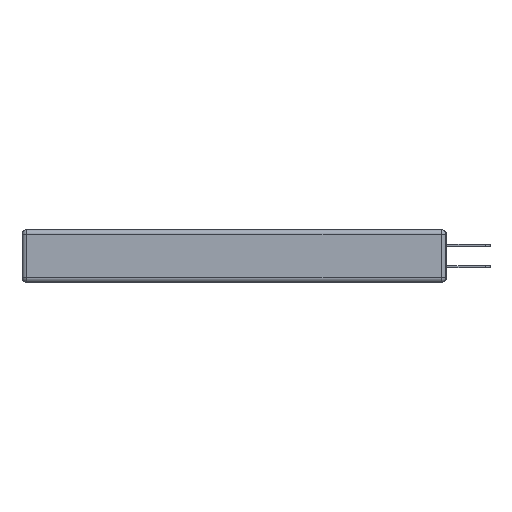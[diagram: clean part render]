
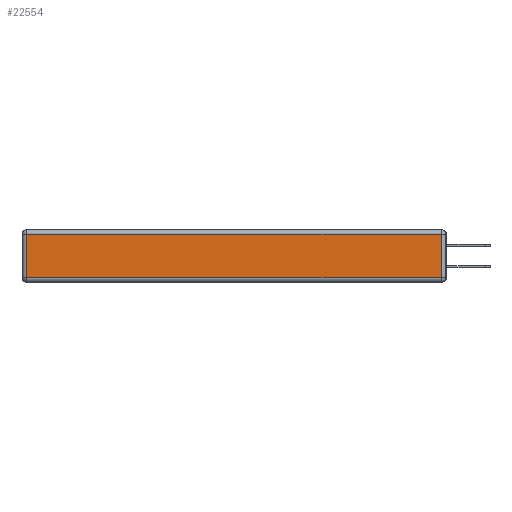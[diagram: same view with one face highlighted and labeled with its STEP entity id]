
A CAD part, left-side view. The second image highlights one B-rep face of the part: STEP entity #22554.
In plain terms, the highlighted planar face has unit normal (-1, 0, 0).
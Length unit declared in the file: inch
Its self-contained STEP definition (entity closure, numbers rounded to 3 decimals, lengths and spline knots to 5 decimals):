
#758 = DIRECTION ( 'NONE',  ( 0., -1., 0. ) ) ;
#1294 = CARTESIAN_POINT ( 'NONE',  ( 0., 2.72, -0.343 ) ) ;
#2915 = VERTEX_POINT ( 'NONE', #11813 ) ;
#3330 = CARTESIAN_POINT ( 'NONE',  ( 0., 0.03, -0.343 ) ) ;
#3584 = CARTESIAN_POINT ( 'NONE',  ( 0., 2.72, -0.313 ) ) ;
#4252 = EDGE_CURVE ( 'NONE', #2915, #4640, #5117, .T. ) ;
#4483 = ORIENTED_EDGE ( 'NONE', *, *, #11383, .T. ) ;
#4640 = VERTEX_POINT ( 'NONE', #8122 ) ;
#5046 = EDGE_LOOP ( 'NONE', ( #4483, #16891, #20012, #7125 ) ) ;
#5117 = LINE ( 'NONE', #3330, #7972 ) ;
#5632 = LINE ( 'NONE', #23146, #7637 ) ;
#5825 = DIRECTION ( 'NONE',  ( -1., 0., 0. ) ) ;
#6559 = CARTESIAN_POINT ( 'NONE',  ( 0., 2.72, -0.03 ) ) ;
#7125 = ORIENTED_EDGE ( 'NONE', *, *, #11200, .T. ) ;
#7637 = VECTOR ( 'NONE', #758, 39.37008 ) ;
#7972 = VECTOR ( 'NONE', #22079, 39.37008 ) ;
#8122 = CARTESIAN_POINT ( 'NONE',  ( 0., 0.03, -0.03 ) ) ;
#8263 = VERTEX_POINT ( 'NONE', #6559 ) ;
#8512 = VECTOR ( 'NONE', #16277, 39.37008 ) ;
#11152 = LINE ( 'NONE', #1294, #8512 ) ;
#11200 = EDGE_CURVE ( 'NONE', #8263, #21469, #11152, .T. ) ;
#11383 = EDGE_CURVE ( 'NONE', #21469, #2915, #5632, .T. ) ;
#11813 = CARTESIAN_POINT ( 'NONE',  ( 0., 0.03, -0.313 ) ) ;
#13420 = PLANE ( 'NONE',  #20109 ) ;
#13977 = FACE_OUTER_BOUND ( 'NONE', #5046, .T. ) ;
#15623 = VECTOR ( 'NONE', #20576, 39.37008 ) ;
#16277 = DIRECTION ( 'NONE',  ( 0., 0., -1. ) ) ;
#16891 = ORIENTED_EDGE ( 'NONE', *, *, #4252, .T. ) ;
#16952 = CARTESIAN_POINT ( 'NONE',  ( 0., 0., -0.343 ) ) ;
#17019 = CARTESIAN_POINT ( 'NONE',  ( 0., 2.75, -0.03 ) ) ;
#17188 = DIRECTION ( 'NONE',  ( 0., 0., 1. ) ) ;
#19715 = EDGE_CURVE ( 'NONE', #4640, #8263, #20642, .T. ) ;
#20012 = ORIENTED_EDGE ( 'NONE', *, *, #19715, .T. ) ;
#20109 = AXIS2_PLACEMENT_3D ( 'NONE', #16952, #5825, #17188 ) ;
#20576 = DIRECTION ( 'NONE',  ( 0., 1., 0. ) ) ;
#20642 = LINE ( 'NONE', #17019, #15623 ) ;
#21469 = VERTEX_POINT ( 'NONE', #3584 ) ;
#22079 = DIRECTION ( 'NONE',  ( 0., 0., 1. ) ) ;
#22554 = ADVANCED_FACE ( 'NONE', ( #13977 ), #13420, .T. ) ;
#23146 = CARTESIAN_POINT ( 'NONE',  ( 0., 0., -0.313 ) ) ;
